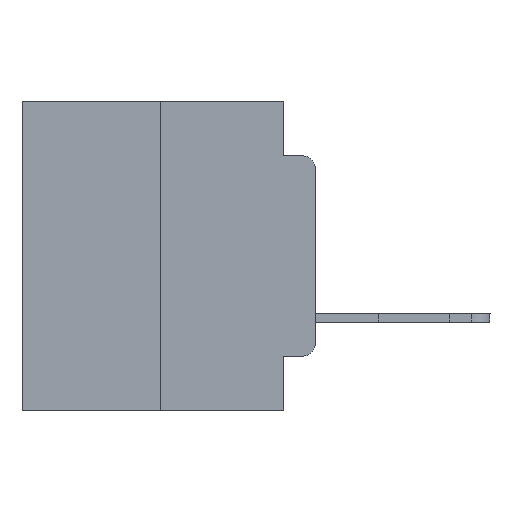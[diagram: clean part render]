
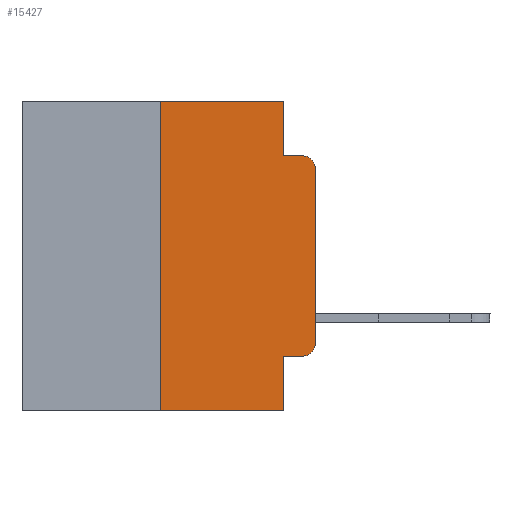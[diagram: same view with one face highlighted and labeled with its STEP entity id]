
A CAD part, left-side view. The second image highlights one B-rep face of the part: STEP entity #15427.
In plain terms, the highlighted planar face has unit normal (-1, 0, 0).
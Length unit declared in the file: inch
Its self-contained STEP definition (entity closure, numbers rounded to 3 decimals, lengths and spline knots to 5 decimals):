
#236 = LINE ( 'NONE', #4306, #2466 ) ;
#368 = CARTESIAN_POINT ( 'NONE',  ( 0., 0.02, -0.3915 ) ) ;
#370 = VECTOR ( 'NONE', #15453, 39.37008 ) ;
#605 = DIRECTION ( 'NONE',  ( 0., 0., -1. ) ) ;
#999 = FACE_OUTER_BOUND ( 'NONE', #3941, .T. ) ;
#1081 = CARTESIAN_POINT ( 'NONE',  ( 0., 0.051, -0.4115 ) ) ;
#1201 = EDGE_CURVE ( 'NONE', #20164, #20904, #236, .T. ) ;
#1660 = VERTEX_POINT ( 'NONE', #2823 ) ;
#2107 = CARTESIAN_POINT ( 'NONE',  ( 0., 0.02, -0.0885 ) ) ;
#2319 = CARTESIAN_POINT ( 'NONE',  ( 0., 0., -0.1085 ) ) ;
#2466 = VECTOR ( 'NONE', #12251, 39.37008 ) ;
#2699 = VERTEX_POINT ( 'NONE', #2107 ) ;
#2811 = DIRECTION ( 'NONE',  ( 0., -1., 0. ) ) ;
#2822 = CIRCLE ( 'NONE', #12809, 0.02 ) ;
#2823 = CARTESIAN_POINT ( 'NONE',  ( 0., 0.25, -0.5 ) ) ;
#2949 = VERTEX_POINT ( 'NONE', #19280 ) ;
#3386 = CARTESIAN_POINT ( 'NONE',  ( 0., 0.051, 0. ) ) ;
#3941 = EDGE_LOOP ( 'NONE', ( #6644, #14553, #17459, #4389, #21116, #15775, #10400, #14600, #13925, #4604 ) ) ;
#4306 = CARTESIAN_POINT ( 'NONE',  ( 0., 0.473, 0. ) ) ;
#4328 = LINE ( 'NONE', #4841, #21228 ) ;
#4389 = ORIENTED_EDGE ( 'NONE', *, *, #7349, .F. ) ;
#4604 = ORIENTED_EDGE ( 'NONE', *, *, #19435, .T. ) ;
#4841 = CARTESIAN_POINT ( 'NONE',  ( 0., 0., 0. ) ) ;
#4909 = LINE ( 'NONE', #18406, #21032 ) ;
#5145 = VECTOR ( 'NONE', #16778, 39.37008 ) ;
#5263 = DIRECTION ( 'NONE',  ( 0., -1., 0. ) ) ;
#5312 = LINE ( 'NONE', #19080, #21428 ) ;
#5342 = LINE ( 'NONE', #25305, #370 ) ;
#5443 = EDGE_CURVE ( 'NONE', #13719, #2699, #9198, .T. ) ;
#5581 = CARTESIAN_POINT ( 'NONE',  ( 0., 0., -0.3915 ) ) ;
#5629 = EDGE_CURVE ( 'NONE', #6957, #13719, #4328, .T. ) ;
#6003 = DIRECTION ( 'NONE',  ( 0., 0., -1. ) ) ;
#6506 = PLANE ( 'NONE',  #11469 ) ;
#6512 = VERTEX_POINT ( 'NONE', #15615 ) ;
#6644 = ORIENTED_EDGE ( 'NONE', *, *, #5629, .T. ) ;
#6957 = VERTEX_POINT ( 'NONE', #5581 ) ;
#7343 = LINE ( 'NONE', #11006, #15199 ) ;
#7349 = EDGE_CURVE ( 'NONE', #20904, #6512, #5312, .T. ) ;
#8249 = CARTESIAN_POINT ( 'NONE',  ( 0., 0.25, 0. ) ) ;
#8723 = DIRECTION ( 'NONE',  ( 1., 0., 0. ) ) ;
#9198 = CIRCLE ( 'NONE', #17491, 0.02 ) ;
#9544 = DIRECTION ( 'NONE',  ( -1., 0., 0. ) ) ;
#9898 = VERTEX_POINT ( 'NONE', #10576 ) ;
#10400 = ORIENTED_EDGE ( 'NONE', *, *, #15936, .T. ) ;
#10576 = CARTESIAN_POINT ( 'NONE',  ( 0., 0.02, -0.4115 ) ) ;
#11006 = CARTESIAN_POINT ( 'NONE',  ( 0., 0.051, -0.4115 ) ) ;
#11011 = EDGE_CURVE ( 'NONE', #24255, #2949, #17166, .T. ) ;
#11469 = AXIS2_PLACEMENT_3D ( 'NONE', #22225, #8723, #605 ) ;
#11972 = DIRECTION ( 'NONE',  ( 0., 0., 1. ) ) ;
#12251 = DIRECTION ( 'NONE',  ( 0., -1., 0. ) ) ;
#12316 = EDGE_CURVE ( 'NONE', #1660, #20164, #23389, .T. ) ;
#12809 = AXIS2_PLACEMENT_3D ( 'NONE', #368, #14063, #6003 ) ;
#13719 = VERTEX_POINT ( 'NONE', #2319 ) ;
#13925 = ORIENTED_EDGE ( 'NONE', *, *, #16439, .T. ) ;
#14063 = DIRECTION ( 'NONE',  ( -1., 0., 0. ) ) ;
#14553 = ORIENTED_EDGE ( 'NONE', *, *, #5443, .T. ) ;
#14600 = ORIENTED_EDGE ( 'NONE', *, *, #11011, .F. ) ;
#14705 = DIRECTION ( 'NONE',  ( 0., 0., 1. ) ) ;
#15199 = VECTOR ( 'NONE', #5263, 39.37008 ) ;
#15245 = DIRECTION ( 'NONE',  ( 0., 0., -1. ) ) ;
#15375 = CARTESIAN_POINT ( 'NONE',  ( 0., 0.02, -0.1085 ) ) ;
#15427 = ADVANCED_FACE ( 'NONE', ( #999 ), #6506, .F. ) ;
#15453 = DIRECTION ( 'NONE',  ( 0., -1., 0. ) ) ;
#15615 = CARTESIAN_POINT ( 'NONE',  ( 0., 0.051, -0.0885 ) ) ;
#15775 = ORIENTED_EDGE ( 'NONE', *, *, #12316, .F. ) ;
#15936 = EDGE_CURVE ( 'NONE', #1660, #2949, #4909, .T. ) ;
#15978 = CARTESIAN_POINT ( 'NONE',  ( 0., 0.25, 0. ) ) ;
#16439 = EDGE_CURVE ( 'NONE', #24255, #9898, #7343, .T. ) ;
#16778 = DIRECTION ( 'NONE',  ( 0., 0., -1. ) ) ;
#17166 = LINE ( 'NONE', #24679, #5145 ) ;
#17459 = ORIENTED_EDGE ( 'NONE', *, *, #20895, .F. ) ;
#17491 = AXIS2_PLACEMENT_3D ( 'NONE', #15375, #9544, #15245 ) ;
#17498 = DIRECTION ( 'NONE',  ( 0., 0., -1. ) ) ;
#18406 = CARTESIAN_POINT ( 'NONE',  ( 0., 0.473, -0.5 ) ) ;
#19080 = CARTESIAN_POINT ( 'NONE',  ( 0., 0.051, 0. ) ) ;
#19280 = CARTESIAN_POINT ( 'NONE',  ( 0., 0.051, -0.5 ) ) ;
#19435 = EDGE_CURVE ( 'NONE', #9898, #6957, #2822, .T. ) ;
#20164 = VERTEX_POINT ( 'NONE', #8249 ) ;
#20895 = EDGE_CURVE ( 'NONE', #6512, #2699, #5342, .T. ) ;
#20904 = VERTEX_POINT ( 'NONE', #3386 ) ;
#21032 = VECTOR ( 'NONE', #2811, 39.37008 ) ;
#21116 = ORIENTED_EDGE ( 'NONE', *, *, #1201, .F. ) ;
#21228 = VECTOR ( 'NONE', #14705, 39.37008 ) ;
#21428 = VECTOR ( 'NONE', #17498, 39.37008 ) ;
#22225 = CARTESIAN_POINT ( 'NONE',  ( 0., 0.473, 0. ) ) ;
#23389 = LINE ( 'NONE', #15978, #24087 ) ;
#24087 = VECTOR ( 'NONE', #11972, 39.37008 ) ;
#24255 = VERTEX_POINT ( 'NONE', #1081 ) ;
#24679 = CARTESIAN_POINT ( 'NONE',  ( 0., 0.051, 0. ) ) ;
#25305 = CARTESIAN_POINT ( 'NONE',  ( 0., 0.051, -0.0885 ) ) ;
